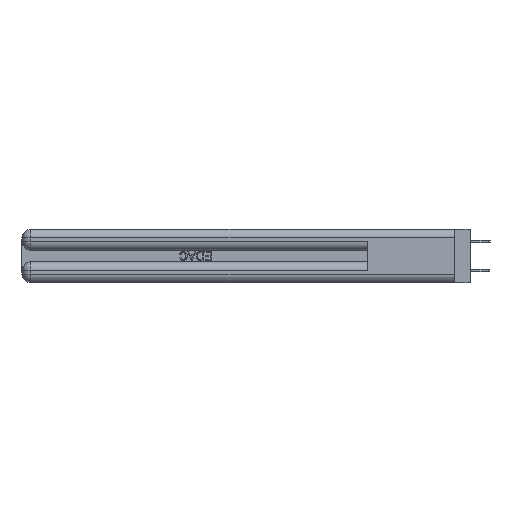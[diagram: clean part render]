
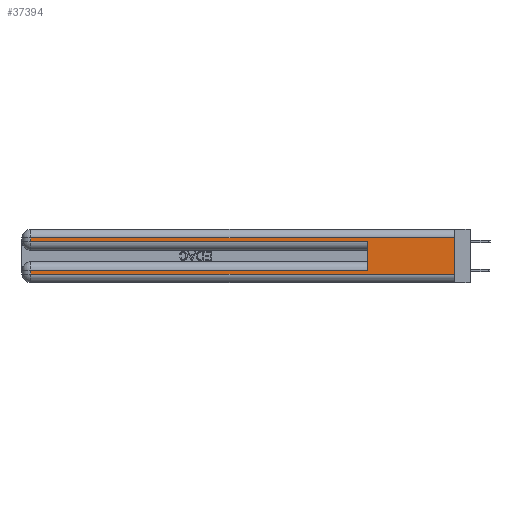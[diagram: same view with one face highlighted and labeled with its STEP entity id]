
A CAD part, left-side view. The second image highlights one B-rep face of the part: STEP entity #37394.
In plain terms, the highlighted planar face has unit normal (-1, 0, 0).
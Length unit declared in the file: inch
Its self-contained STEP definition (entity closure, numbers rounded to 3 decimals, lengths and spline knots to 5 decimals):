
#1624 = VECTOR ( 'NONE', #32651, 39.37008 ) ;
#1702 = DIRECTION ( 'NONE',  ( 0., -1., 0. ) ) ;
#2379 = EDGE_LOOP ( 'NONE', ( #15084, #20221, #48911, #48110, #26859, #26048, #42323, #14780 ) ) ;
#5283 = VERTEX_POINT ( 'NONE', #11746 ) ;
#6418 = LINE ( 'NONE', #33253, #24409 ) ;
#7737 = FACE_OUTER_BOUND ( 'NONE', #2379, .T. ) ;
#7997 = DIRECTION ( 'NONE',  ( 1., 0., 0. ) ) ;
#8264 = DIRECTION ( 'NONE',  ( 0., 0., -1. ) ) ;
#8349 = DIRECTION ( 'NONE',  ( 0., 0., -1. ) ) ;
#9239 = LINE ( 'NONE', #25363, #19001 ) ;
#9472 = LINE ( 'NONE', #21189, #1624 ) ;
#10792 = DIRECTION ( 'NONE',  ( 0., 1., 0. ) ) ;
#11746 = CARTESIAN_POINT ( 'NONE',  ( 0., 2.94, 0.06 ) ) ;
#11811 = EDGE_CURVE ( 'NONE', #39055, #23922, #9472, .T. ) ;
#12520 = CARTESIAN_POINT ( 'NONE',  ( 0., 0., 0.31 ) ) ;
#13286 = CARTESIAN_POINT ( 'NONE',  ( 0., 2.94, 0.31 ) ) ;
#14624 = CARTESIAN_POINT ( 'NONE',  ( 0., 2.94, 0.285 ) ) ;
#14780 = ORIENTED_EDGE ( 'NONE', *, *, #45628, .T. ) ;
#14998 = LINE ( 'NONE', #18898, #18504 ) ;
#15084 = ORIENTED_EDGE ( 'NONE', *, *, #48607, .F. ) ;
#17522 = DIRECTION ( 'NONE',  ( 0., -1., 0. ) ) ;
#17763 = LINE ( 'NONE', #33653, #34949 ) ;
#18504 = VECTOR ( 'NONE', #30862, 39.37008 ) ;
#18898 = CARTESIAN_POINT ( 'NONE',  ( 0., 0., 0.37 ) ) ;
#19001 = VECTOR ( 'NONE', #1702, 39.37008 ) ;
#19701 = CARTESIAN_POINT ( 'NONE',  ( 0., 0., 0.06 ) ) ;
#19721 = CARTESIAN_POINT ( 'NONE',  ( 0., 2.94, 0.37 ) ) ;
#20221 = ORIENTED_EDGE ( 'NONE', *, *, #11811, .T. ) ;
#21189 = CARTESIAN_POINT ( 'NONE',  ( 0., 0., 0.31 ) ) ;
#21843 = VERTEX_POINT ( 'NONE', #19701 ) ;
#23922 = VERTEX_POINT ( 'NONE', #13286 ) ;
#24274 = EDGE_CURVE ( 'NONE', #36429, #5283, #32716, .T. ) ;
#24409 = VECTOR ( 'NONE', #49106, 39.37008 ) ;
#24480 = CARTESIAN_POINT ( 'NONE',  ( 0., 0., 0.085 ) ) ;
#25363 = CARTESIAN_POINT ( 'NONE',  ( 0., 0., 0.285 ) ) ;
#25695 = VECTOR ( 'NONE', #8264, 39.37008 ) ;
#26048 = ORIENTED_EDGE ( 'NONE', *, *, #29830, .T. ) ;
#26469 = CARTESIAN_POINT ( 'NONE',  ( 0., 0.6, 0.285 ) ) ;
#26859 = ORIENTED_EDGE ( 'NONE', *, *, #51113, .F. ) ;
#27197 = LINE ( 'NONE', #24480, #49435 ) ;
#29830 = EDGE_CURVE ( 'NONE', #47211, #36429, #27197, .T. ) ;
#30862 = DIRECTION ( 'NONE',  ( 0., 0., -1. ) ) ;
#32320 = CARTESIAN_POINT ( 'NONE',  ( 0., 2.94, 0.085 ) ) ;
#32651 = DIRECTION ( 'NONE',  ( 0., 1., 0. ) ) ;
#32716 = LINE ( 'NONE', #19721, #25695 ) ;
#33253 = CARTESIAN_POINT ( 'NONE',  ( 0., 0.6, 0.145 ) ) ;
#33627 = VERTEX_POINT ( 'NONE', #14624 ) ;
#33653 = CARTESIAN_POINT ( 'NONE',  ( 0., 0., 0.06 ) ) ;
#34937 = VECTOR ( 'NONE', #8349, 39.37008 ) ;
#34949 = VECTOR ( 'NONE', #17522, 39.37008 ) ;
#35161 = LINE ( 'NONE', #44008, #34937 ) ;
#35849 = PLANE ( 'NONE',  #48944 ) ;
#36429 = VERTEX_POINT ( 'NONE', #32320 ) ;
#37394 = ADVANCED_FACE ( 'NONE', ( #7737 ), #35849, .F. ) ;
#38147 = EDGE_CURVE ( 'NONE', #33627, #49833, #9239, .T. ) ;
#39055 = VERTEX_POINT ( 'NONE', #12520 ) ;
#40233 = EDGE_CURVE ( 'NONE', #23922, #33627, #35161, .T. ) ;
#42323 = ORIENTED_EDGE ( 'NONE', *, *, #24274, .T. ) ;
#43156 = CARTESIAN_POINT ( 'NONE',  ( 0., 0., 0.37 ) ) ;
#43914 = DIRECTION ( 'NONE',  ( 0., 0., -1. ) ) ;
#44008 = CARTESIAN_POINT ( 'NONE',  ( 0., 2.94, 0.37 ) ) ;
#45628 = EDGE_CURVE ( 'NONE', #5283, #21843, #17763, .T. ) ;
#46224 = CARTESIAN_POINT ( 'NONE',  ( 0., 0.6, 0.085 ) ) ;
#47211 = VERTEX_POINT ( 'NONE', #46224 ) ;
#48110 = ORIENTED_EDGE ( 'NONE', *, *, #38147, .T. ) ;
#48607 = EDGE_CURVE ( 'NONE', #39055, #21843, #14998, .T. ) ;
#48911 = ORIENTED_EDGE ( 'NONE', *, *, #40233, .T. ) ;
#48944 = AXIS2_PLACEMENT_3D ( 'NONE', #43156, #7997, #43914 ) ;
#49106 = DIRECTION ( 'NONE',  ( 0., 0., 1. ) ) ;
#49435 = VECTOR ( 'NONE', #10792, 39.37008 ) ;
#49833 = VERTEX_POINT ( 'NONE', #26469 ) ;
#51113 = EDGE_CURVE ( 'NONE', #47211, #49833, #6418, .T. ) ;
